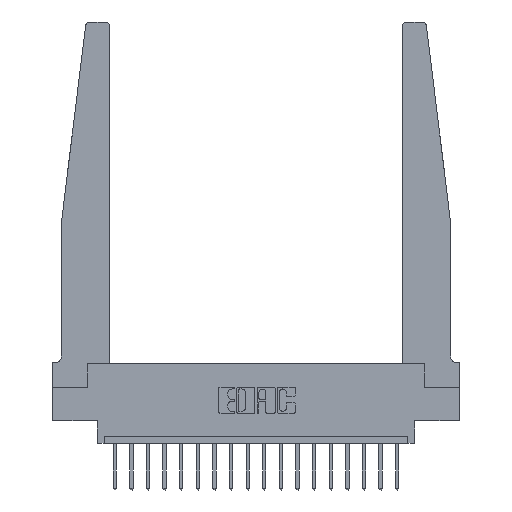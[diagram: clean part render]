
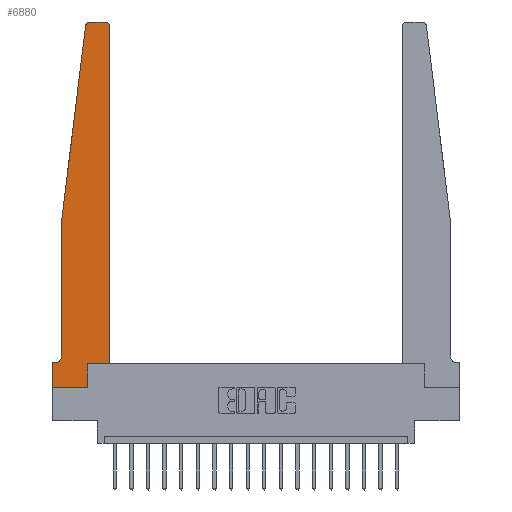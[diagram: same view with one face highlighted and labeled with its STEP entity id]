
A CAD part, top view. The second image highlights one B-rep face of the part: STEP entity #6880.
In plain terms, the highlighted planar face has unit normal (0, 0, 1).
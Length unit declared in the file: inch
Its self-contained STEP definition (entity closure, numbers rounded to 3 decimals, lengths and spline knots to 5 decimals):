
#540 = CARTESIAN_POINT ( 'NONE',  ( 0., 0., 0.37 ) ) ;
#614 = LINE ( 'NONE', #14483, #9593 ) ;
#1094 = EDGE_LOOP ( 'NONE', ( #11039, #14458, #10360, #3231, #2030, #13109, #3213, #12916, #4922, #7096, #11909, #6562 ) ) ;
#1399 = CARTESIAN_POINT ( 'NONE',  ( 0.2605, 0., 0.37 ) ) ;
#1906 = LINE ( 'NONE', #18706, #7343 ) ;
#2030 = ORIENTED_EDGE ( 'NONE', *, *, #6501, .T. ) ;
#2100 = CARTESIAN_POINT ( 'NONE',  ( 0.425, 2.72, 0.37 ) ) ;
#2109 = VERTEX_POINT ( 'NONE', #3779 ) ;
#2132 = DIRECTION ( 'NONE',  ( 1., 0., 0. ) ) ;
#2172 = DIRECTION ( 'NONE',  ( 0., 0., 1. ) ) ;
#2453 = VERTEX_POINT ( 'NONE', #3344 ) ;
#2460 = DIRECTION ( 'NONE',  ( 1., 0., 0. ) ) ;
#3213 = ORIENTED_EDGE ( 'NONE', *, *, #6715, .T. ) ;
#3231 = ORIENTED_EDGE ( 'NONE', *, *, #13681, .T. ) ;
#3344 = CARTESIAN_POINT ( 'NONE',  ( 0., 0.1875, 0.37 ) ) ;
#3488 = VERTEX_POINT ( 'NONE', #1399 ) ;
#3632 = CARTESIAN_POINT ( 'NONE',  ( 0., 0., 0.37 ) ) ;
#3676 = PLANE ( 'NONE',  #17584 ) ;
#3761 = CARTESIAN_POINT ( 'NONE',  ( 0.24675, 2.72367, 0.37 ) ) ;
#3779 = CARTESIAN_POINT ( 'NONE',  ( 0.065, 1.25, 0.37 ) ) ;
#4049 = DIRECTION ( 'NONE',  ( 0., 0., 1. ) ) ;
#4485 = DIRECTION ( 'NONE',  ( 0., 1., 0. ) ) ;
#4671 = EDGE_CURVE ( 'NONE', #17730, #9138, #10185, .T. ) ;
#4715 = DIRECTION ( 'NONE',  ( 0., 0., -1. ) ) ;
#4886 = CARTESIAN_POINT ( 'NONE',  ( 0.27653, 2.75, 0.37 ) ) ;
#4922 = ORIENTED_EDGE ( 'NONE', *, *, #13107, .T. ) ;
#4998 = VERTEX_POINT ( 'NONE', #7930 ) ;
#5017 = DIRECTION ( 'NONE',  ( -0.122, -0.992, 0. ) ) ;
#5466 = FACE_OUTER_BOUND ( 'NONE', #1094, .T. ) ;
#5675 = VERTEX_POINT ( 'NONE', #17251 ) ;
#5883 = VECTOR ( 'NONE', #10960, 39.37008 ) ;
#6417 = EDGE_CURVE ( 'NONE', #9138, #2109, #1906, .T. ) ;
#6501 = EDGE_CURVE ( 'NONE', #18117, #4998, #8331, .T. ) ;
#6562 = ORIENTED_EDGE ( 'NONE', *, *, #9957, .T. ) ;
#6715 = EDGE_CURVE ( 'NONE', #2453, #15848, #614, .T. ) ;
#6872 = CARTESIAN_POINT ( 'NONE',  ( 0., 0.1875, 0.37 ) ) ;
#6880 = ADVANCED_FACE ( 'NONE', ( #5466 ), #3676, .T. ) ;
#6915 = DIRECTION ( 'NONE',  ( 0., -1., 0. ) ) ;
#6933 = LINE ( 'NONE', #540, #11598 ) ;
#7096 = ORIENTED_EDGE ( 'NONE', *, *, #13577, .T. ) ;
#7343 = VECTOR ( 'NONE', #5017, 39.37008 ) ;
#7600 = CARTESIAN_POINT ( 'NONE',  ( 0.2605, 0.18, 0.37 ) ) ;
#7930 = CARTESIAN_POINT ( 'NONE',  ( 0.015, 0.1875, 0.37 ) ) ;
#8075 = CARTESIAN_POINT ( 'NONE',  ( 0.2605, 0.18, 0.37 ) ) ;
#8331 = CIRCLE ( 'NONE', #11806, 0.05 ) ;
#8815 = CARTESIAN_POINT ( 'NONE',  ( 0.065, 1.25, 0.37 ) ) ;
#8916 = VERTEX_POINT ( 'NONE', #11835 ) ;
#9138 = VERTEX_POINT ( 'NONE', #3761 ) ;
#9593 = VECTOR ( 'NONE', #6915, 39.37008 ) ;
#9957 = EDGE_CURVE ( 'NONE', #11383, #8916, #11279, .T. ) ;
#10185 = CIRCLE ( 'NONE', #12732, 0.03 ) ;
#10345 = VECTOR ( 'NONE', #14251, 39.37008 ) ;
#10355 = DIRECTION ( 'NONE',  ( -1., 0., 0. ) ) ;
#10360 = ORIENTED_EDGE ( 'NONE', *, *, #6417, .T. ) ;
#10664 = LINE ( 'NONE', #16763, #5883 ) ;
#10762 = CARTESIAN_POINT ( 'NONE',  ( 0.425, 0.18, 0.37 ) ) ;
#10960 = DIRECTION ( 'NONE',  ( -1., 0., 0. ) ) ;
#10992 = DIRECTION ( 'NONE',  ( -1., 0., 0. ) ) ;
#11039 = ORIENTED_EDGE ( 'NONE', *, *, #13007, .T. ) ;
#11279 = CIRCLE ( 'NONE', #11900, 0.03 ) ;
#11290 = DIRECTION ( 'NONE',  ( 0., 0., 1. ) ) ;
#11338 = VECTOR ( 'NONE', #19509, 39.37008 ) ;
#11383 = VERTEX_POINT ( 'NONE', #2100 ) ;
#11598 = VECTOR ( 'NONE', #2132, 39.37008 ) ;
#11806 = AXIS2_PLACEMENT_3D ( 'NONE', #15700, #4715, #10992 ) ;
#11835 = CARTESIAN_POINT ( 'NONE',  ( 0.395, 2.75, 0.37 ) ) ;
#11840 = CARTESIAN_POINT ( 'NONE',  ( 0.065, 0.1875, 0.37 ) ) ;
#11900 = AXIS2_PLACEMENT_3D ( 'NONE', #17203, #11290, #12582 ) ;
#11909 = ORIENTED_EDGE ( 'NONE', *, *, #15292, .T. ) ;
#12188 = EDGE_CURVE ( 'NONE', #15848, #3488, #6933, .T. ) ;
#12260 = VECTOR ( 'NONE', #18648, 39.37008 ) ;
#12489 = VERTEX_POINT ( 'NONE', #7600 ) ;
#12528 = LINE ( 'NONE', #18549, #12260 ) ;
#12582 = DIRECTION ( 'NONE',  ( 1., 0., 0. ) ) ;
#12732 = AXIS2_PLACEMENT_3D ( 'NONE', #14718, #4049, #19341 ) ;
#12916 = ORIENTED_EDGE ( 'NONE', *, *, #12188, .T. ) ;
#13007 = EDGE_CURVE ( 'NONE', #8916, #17730, #10664, .T. ) ;
#13107 = EDGE_CURVE ( 'NONE', #3488, #12489, #15570, .T. ) ;
#13109 = ORIENTED_EDGE ( 'NONE', *, *, #16759, .T. ) ;
#13432 = LINE ( 'NONE', #11840, #15579 ) ;
#13577 = EDGE_CURVE ( 'NONE', #12489, #5675, #12528, .T. ) ;
#13681 = EDGE_CURVE ( 'NONE', #2109, #18117, #17913, .T. ) ;
#14251 = DIRECTION ( 'NONE',  ( 0., 1., 0. ) ) ;
#14458 = ORIENTED_EDGE ( 'NONE', *, *, #4671, .T. ) ;
#14483 = CARTESIAN_POINT ( 'NONE',  ( 0., 0., 0.37 ) ) ;
#14718 = CARTESIAN_POINT ( 'NONE',  ( 0.27653, 2.72, 0.37 ) ) ;
#15292 = EDGE_CURVE ( 'NONE', #5675, #11383, #18567, .T. ) ;
#15570 = LINE ( 'NONE', #8075, #10345 ) ;
#15579 = VECTOR ( 'NONE', #10355, 39.37008 ) ;
#15700 = CARTESIAN_POINT ( 'NONE',  ( 0.015, 0.2375, 0.37 ) ) ;
#15848 = VERTEX_POINT ( 'NONE', #3632 ) ;
#16759 = EDGE_CURVE ( 'NONE', #4998, #2453, #13432, .T. ) ;
#16763 = CARTESIAN_POINT ( 'NONE',  ( 0.25, 2.75, 0.37 ) ) ;
#17203 = CARTESIAN_POINT ( 'NONE',  ( 0.395, 2.72, 0.37 ) ) ;
#17251 = CARTESIAN_POINT ( 'NONE',  ( 0.425, 0.18, 0.37 ) ) ;
#17584 = AXIS2_PLACEMENT_3D ( 'NONE', #6872, #2172, #2460 ) ;
#17644 = CARTESIAN_POINT ( 'NONE',  ( 0.065, 0.2375, 0.37 ) ) ;
#17730 = VERTEX_POINT ( 'NONE', #4886 ) ;
#17773 = VECTOR ( 'NONE', #4485, 39.37008 ) ;
#17913 = LINE ( 'NONE', #8815, #11338 ) ;
#18117 = VERTEX_POINT ( 'NONE', #17644 ) ;
#18549 = CARTESIAN_POINT ( 'NONE',  ( 0.425, 0.18, 0.37 ) ) ;
#18567 = LINE ( 'NONE', #10762, #17773 ) ;
#18648 = DIRECTION ( 'NONE',  ( 1., 0., 0. ) ) ;
#18706 = CARTESIAN_POINT ( 'NONE',  ( 0.065, 1.25, 0.37 ) ) ;
#19341 = DIRECTION ( 'NONE',  ( 1., 0., 0. ) ) ;
#19509 = DIRECTION ( 'NONE',  ( 0., -1., 0. ) ) ;
